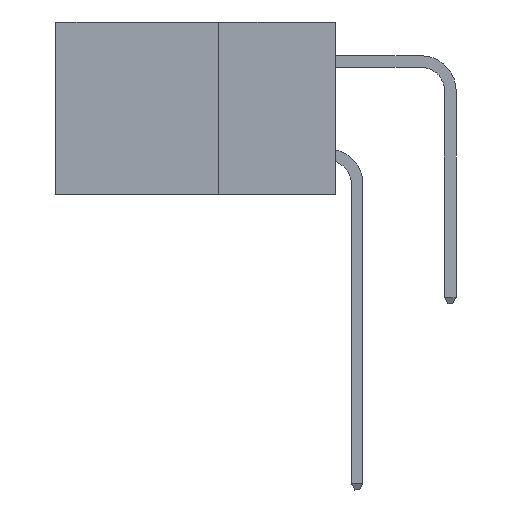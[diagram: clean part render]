
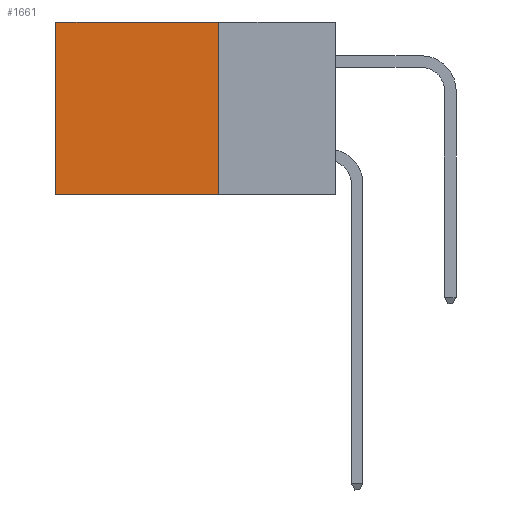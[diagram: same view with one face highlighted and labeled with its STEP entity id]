
A CAD part, left-side view. The second image highlights one B-rep face of the part: STEP entity #1661.
In plain terms, the highlighted planar face has unit normal (-1, 0, 0).
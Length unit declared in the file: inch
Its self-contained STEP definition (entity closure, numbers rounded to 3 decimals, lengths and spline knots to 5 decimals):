
#281 = LINE ( 'NONE', #18290, #28072 ) ;
#1025 = VERTEX_POINT ( 'NONE', #29448 ) ;
#1661 = ADVANCED_FACE ( 'NONE', ( #23335 ), #16974, .F. ) ;
#3668 = ORIENTED_EDGE ( 'NONE', *, *, #35412, .T. ) ;
#5923 = EDGE_CURVE ( 'NONE', #35794, #22022, #14675, .T. ) ;
#6824 = VECTOR ( 'NONE', #11840, 39.37008 ) ;
#7718 = VECTOR ( 'NONE', #12460, 39.37008 ) ;
#8363 = CARTESIAN_POINT ( 'NONE',  ( 0.2875, 0.25, 0. ) ) ;
#10227 = EDGE_CURVE ( 'NONE', #15823, #35794, #281, .T. ) ;
#11139 = DIRECTION ( 'NONE',  ( 1., 0., 0. ) ) ;
#11768 = VECTOR ( 'NONE', #12992, 39.37008 ) ;
#11840 = DIRECTION ( 'NONE',  ( 0., 1., 0. ) ) ;
#12460 = DIRECTION ( 'NONE',  ( 0., 1., 0. ) ) ;
#12992 = DIRECTION ( 'NONE',  ( 0., 0., -1. ) ) ;
#14132 = EDGE_CURVE ( 'NONE', #1025, #22022, #32135, .T. ) ;
#14675 = LINE ( 'NONE', #32319, #7718 ) ;
#15823 = VERTEX_POINT ( 'NONE', #31169 ) ;
#16723 = DIRECTION ( 'NONE',  ( 0., 0., -1. ) ) ;
#16913 = ORIENTED_EDGE ( 'NONE', *, *, #5923, .F. ) ;
#16974 = PLANE ( 'NONE',  #27141 ) ;
#18290 = CARTESIAN_POINT ( 'NONE',  ( 0.2875, 0.25, 0. ) ) ;
#21228 = CARTESIAN_POINT ( 'NONE',  ( 0.2875, 0.6, 0. ) ) ;
#21606 = LINE ( 'NONE', #34367, #6824 ) ;
#22022 = VERTEX_POINT ( 'NONE', #32150 ) ;
#23335 = FACE_OUTER_BOUND ( 'NONE', #25758, .T. ) ;
#25758 = EDGE_LOOP ( 'NONE', ( #27706, #16913, #26258, #3668 ) ) ;
#26258 = ORIENTED_EDGE ( 'NONE', *, *, #10227, .F. ) ;
#27141 = AXIS2_PLACEMENT_3D ( 'NONE', #8363, #11139, #16723 ) ;
#27706 = ORIENTED_EDGE ( 'NONE', *, *, #14132, .T. ) ;
#28072 = VECTOR ( 'NONE', #35246, 39.37008 ) ;
#28681 = CARTESIAN_POINT ( 'NONE',  ( 0.2875, 0.25, -0.37 ) ) ;
#29448 = CARTESIAN_POINT ( 'NONE',  ( 0.2875, 0.6, 0. ) ) ;
#31169 = CARTESIAN_POINT ( 'NONE',  ( 0.2875, 0.25, 0. ) ) ;
#32135 = LINE ( 'NONE', #21228, #11768 ) ;
#32150 = CARTESIAN_POINT ( 'NONE',  ( 0.2875, 0.6, -0.37 ) ) ;
#32319 = CARTESIAN_POINT ( 'NONE',  ( 0.2875, 0.25, -0.37 ) ) ;
#34367 = CARTESIAN_POINT ( 'NONE',  ( 0.2875, 0.25, 0. ) ) ;
#35246 = DIRECTION ( 'NONE',  ( 0., 0., -1. ) ) ;
#35412 = EDGE_CURVE ( 'NONE', #15823, #1025, #21606, .T. ) ;
#35794 = VERTEX_POINT ( 'NONE', #28681 ) ;
